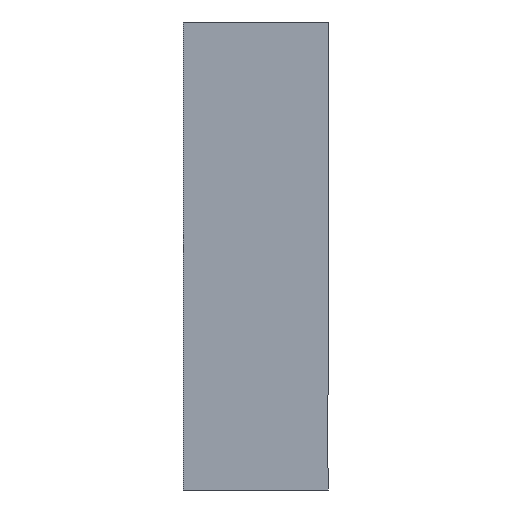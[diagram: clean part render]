
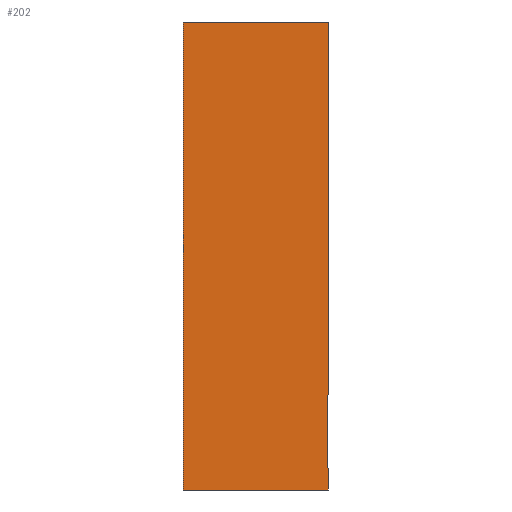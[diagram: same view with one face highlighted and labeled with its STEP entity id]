
A CAD part, front view. The second image highlights one B-rep face of the part: STEP entity #202.
In plain terms, the highlighted planar face has unit normal (0, -1, 0).
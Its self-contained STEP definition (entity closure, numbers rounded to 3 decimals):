
#73=CARTESIAN_POINT('',(7.906,2.8,7.));
#74=VERTEX_POINT('',#73);
#83=CARTESIAN_POINT('',(2.333,2.8,7.));
#84=VERTEX_POINT('',#83);
#85=CARTESIAN_POINT('',(2.333,2.8,7.));
#86=DIRECTION('',(1.0,0.0,0.0));
#87=VECTOR('',#86,5.573);
#88=LINE('',#85,#87);
#89=EDGE_CURVE('',#84,#74,#88,.T.);
#122=CARTESIAN_POINT('',(2.333,2.8,25.0));
#123=VERTEX_POINT('',#122);
#124=CARTESIAN_POINT('',(2.333,2.8,7.));
#125=DIRECTION('',(0.0,0.0,1.0));
#126=VECTOR('',#125,18.0);
#127=LINE('',#124,#126);
#128=EDGE_CURVE('',#84,#123,#127,.T.);
#163=CARTESIAN_POINT('',(5.133,2.8,0.0));
#164=DIRECTION('',(0.0,1.0,0.0));
#165=DIRECTION('',(-1.0,0.0,0.0));
#166=AXIS2_PLACEMENT_3D('',#163,#164,#165);
#167=PLANE('',#166);
#168=ORIENTED_EDGE('',*,*,#89,.T.);
#169=CARTESIAN_POINT('',(7.89,2.8,10.428));
#170=VERTEX_POINT('',#169);
#171=CARTESIAN_POINT('',(7.89,2.8,10.428));
#172=DIRECTION('',(0.005,0.0,-1.));
#173=VECTOR('',#172,3.428);
#174=LINE('',#171,#173);
#175=EDGE_CURVE('',#170,#74,#174,.T.);
#176=ORIENTED_EDGE('',*,*,#175,.F.);
#177=CARTESIAN_POINT('',(7.933,2.8,11.186));
#178=VERTEX_POINT('',#177);
#179=CARTESIAN_POINT('',(7.933,2.8,11.186));
#180=DIRECTION('',(-0.057,0.0,-0.998));
#181=VECTOR('',#180,0.76);
#182=LINE('',#179,#181);
#183=EDGE_CURVE('',#178,#170,#182,.T.);
#184=ORIENTED_EDGE('',*,*,#183,.F.);
#185=CARTESIAN_POINT('',(7.933,2.8,25.0));
#186=VERTEX_POINT('',#185);
#187=CARTESIAN_POINT('',(7.933,2.8,11.186));
#188=DIRECTION('',(0.0,0.0,1.0));
#189=VECTOR('',#188,13.814);
#190=LINE('',#187,#189);
#191=EDGE_CURVE('',#178,#186,#190,.T.);
#192=ORIENTED_EDGE('',*,*,#191,.T.);
#193=CARTESIAN_POINT('',(7.933,2.8,25.0));
#194=DIRECTION('',(-1.0,0.0,0.0));
#195=VECTOR('',#194,5.6);
#196=LINE('',#193,#195);
#197=EDGE_CURVE('',#186,#123,#196,.T.);
#198=ORIENTED_EDGE('',*,*,#197,.T.);
#199=ORIENTED_EDGE('',*,*,#128,.F.);
#200=EDGE_LOOP('',(#168,#176,#184,#192,#198,#199));
#201=FACE_OUTER_BOUND('',#200,.T.);
#202=ADVANCED_FACE('',(#201),#167,.F.);
